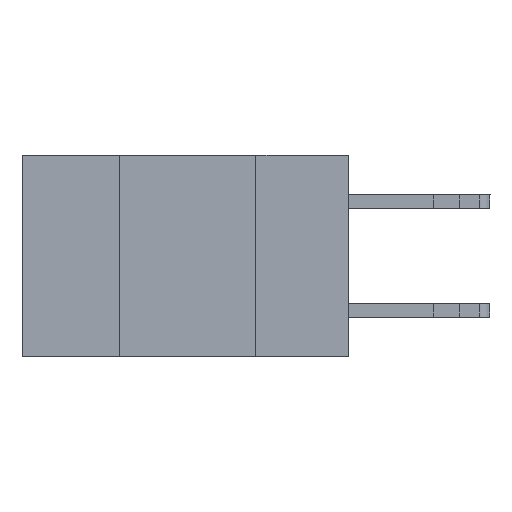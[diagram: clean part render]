
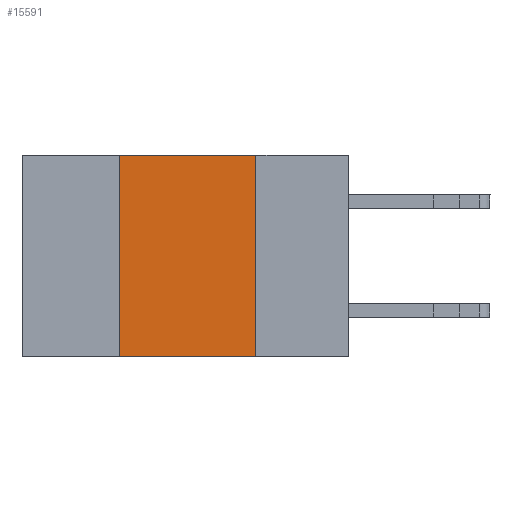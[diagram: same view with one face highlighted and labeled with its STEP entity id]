
A CAD part, left-side view. The second image highlights one B-rep face of the part: STEP entity #15591.
In plain terms, the highlighted planar face has unit normal (-1, 0, 0).
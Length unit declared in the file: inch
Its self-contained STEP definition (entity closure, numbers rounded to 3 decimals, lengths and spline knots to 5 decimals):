
#15 = EDGE_CURVE ( 'NONE', #297, #1578, #13066, .T. ) ;
#297 = VERTEX_POINT ( 'NONE', #15035 ) ;
#544 = ORIENTED_EDGE ( 'NONE', *, *, #15394, .F. ) ;
#795 = CARTESIAN_POINT ( 'NONE',  ( 0., 0.17, -0.37 ) ) ;
#1501 = LINE ( 'NONE', #13414, #3524 ) ;
#1578 = VERTEX_POINT ( 'NONE', #795 ) ;
#1666 = ORIENTED_EDGE ( 'NONE', *, *, #3157, .F. ) ;
#2241 = VERTEX_POINT ( 'NONE', #7816 ) ;
#2904 = AXIS2_PLACEMENT_3D ( 'NONE', #14325, #16101, #10418 ) ;
#3157 = EDGE_CURVE ( 'NONE', #297, #9654, #6229, .T. ) ;
#3524 = VECTOR ( 'NONE', #12107, 39.37008 ) ;
#6229 = LINE ( 'NONE', #10228, #10233 ) ;
#6933 = CARTESIAN_POINT ( 'NONE',  ( 0., 0.6, 0. ) ) ;
#7717 = PLANE ( 'NONE',  #2904 ) ;
#7816 = CARTESIAN_POINT ( 'NONE',  ( 0., 0.17, 0. ) ) ;
#7825 = ORIENTED_EDGE ( 'NONE', *, *, #13601, .F. ) ;
#8107 = ORIENTED_EDGE ( 'NONE', *, *, #15, .T. ) ;
#9654 = VERTEX_POINT ( 'NONE', #12470 ) ;
#10228 = CARTESIAN_POINT ( 'NONE',  ( 0., 0.42, 0. ) ) ;
#10233 = VECTOR ( 'NONE', #15513, 39.37008 ) ;
#10295 = EDGE_LOOP ( 'NONE', ( #7825, #544, #1666, #8107 ) ) ;
#10418 = DIRECTION ( 'NONE',  ( 0., 0., -1. ) ) ;
#12107 = DIRECTION ( 'NONE',  ( 0., 0., -1. ) ) ;
#12114 = VECTOR ( 'NONE', #14621, 39.37008 ) ;
#12242 = DIRECTION ( 'NONE',  ( 0., -1., 0. ) ) ;
#12470 = CARTESIAN_POINT ( 'NONE',  ( 0., 0.42, 0. ) ) ;
#13066 = LINE ( 'NONE', #14363, #12114 ) ;
#13414 = CARTESIAN_POINT ( 'NONE',  ( 0., 0.17, 0. ) ) ;
#13453 = VECTOR ( 'NONE', #12242, 39.37008 ) ;
#13601 = EDGE_CURVE ( 'NONE', #2241, #1578, #1501, .T. ) ;
#14239 = FACE_OUTER_BOUND ( 'NONE', #10295, .T. ) ;
#14325 = CARTESIAN_POINT ( 'NONE',  ( 0., 0.6, 0. ) ) ;
#14363 = CARTESIAN_POINT ( 'NONE',  ( 0., 0.6, -0.37 ) ) ;
#14621 = DIRECTION ( 'NONE',  ( 0., -1., 0. ) ) ;
#14854 = LINE ( 'NONE', #6933, #13453 ) ;
#15035 = CARTESIAN_POINT ( 'NONE',  ( 0., 0.42, -0.37 ) ) ;
#15394 = EDGE_CURVE ( 'NONE', #9654, #2241, #14854, .T. ) ;
#15513 = DIRECTION ( 'NONE',  ( 0., 0., 1. ) ) ;
#15591 = ADVANCED_FACE ( 'NONE', ( #14239 ), #7717, .F. ) ;
#16101 = DIRECTION ( 'NONE',  ( 1., 0., 0. ) ) ;
